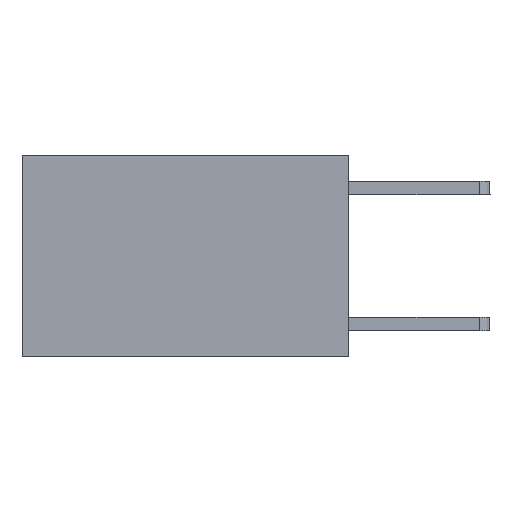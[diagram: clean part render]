
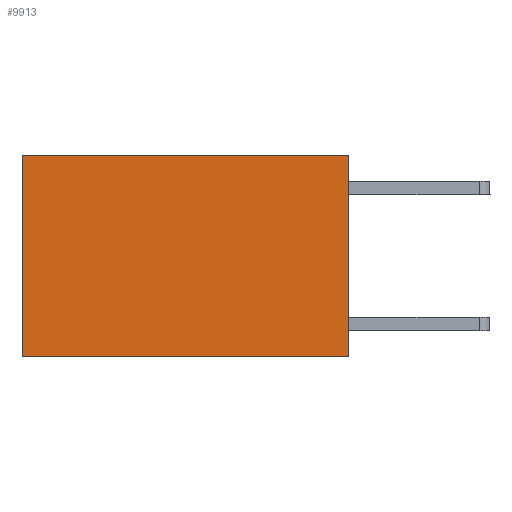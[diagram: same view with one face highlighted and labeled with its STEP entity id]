
A CAD part, left-side view. The second image highlights one B-rep face of the part: STEP entity #9913.
In plain terms, the highlighted planar face has unit normal (-1, 0, 0).
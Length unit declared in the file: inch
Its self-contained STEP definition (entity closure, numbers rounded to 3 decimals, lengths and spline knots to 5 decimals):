
#93 = LINE ( 'NONE', #1786, #122 ) ;
#122 = VECTOR ( 'NONE', #9171, 39.37008 ) ;
#345 = EDGE_CURVE ( 'NONE', #6390, #7943, #980, .T. ) ;
#445 = EDGE_CURVE ( 'NONE', #7943, #3313, #699, .T. ) ;
#623 = EDGE_CURVE ( 'NONE', #8956, #3313, #93, .T. ) ;
#664 = VECTOR ( 'NONE', #1453, 39.37008 ) ;
#699 = LINE ( 'NONE', #6083, #664 ) ;
#959 = VECTOR ( 'NONE', #5688, 39.37008 ) ;
#980 = LINE ( 'NONE', #7719, #959 ) ;
#1453 = DIRECTION ( 'NONE',  ( 0., 1., 0. ) ) ;
#1756 = CARTESIAN_POINT ( 'NONE',  ( 0.2625, 0.6, -0.37 ) ) ;
#1786 = CARTESIAN_POINT ( 'NONE',  ( 0.2625, 0.6, 0. ) ) ;
#2009 = AXIS2_PLACEMENT_3D ( 'NONE', #7611, #9934, #5160 ) ;
#2753 = ORIENTED_EDGE ( 'NONE', *, *, #345, .F. ) ;
#3242 = ORIENTED_EDGE ( 'NONE', *, *, #623, .T. ) ;
#3313 = VERTEX_POINT ( 'NONE', #1756 ) ;
#4189 = DIRECTION ( 'NONE',  ( 0., 1., 0. ) ) ;
#4450 = ORIENTED_EDGE ( 'NONE', *, *, #5101, .T. ) ;
#5101 = EDGE_CURVE ( 'NONE', #6390, #8956, #8676, .T. ) ;
#5160 = DIRECTION ( 'NONE',  ( 0., 0., -1. ) ) ;
#5546 = CARTESIAN_POINT ( 'NONE',  ( 0.2625, 0., -0.37 ) ) ;
#5688 = DIRECTION ( 'NONE',  ( 0., 0., -1. ) ) ;
#6083 = CARTESIAN_POINT ( 'NONE',  ( 0.2625, 0., -0.37 ) ) ;
#6390 = VERTEX_POINT ( 'NONE', #10628 ) ;
#7322 = CARTESIAN_POINT ( 'NONE',  ( 0.2625, 0.6, 0. ) ) ;
#7611 = CARTESIAN_POINT ( 'NONE',  ( 0.2625, 0., 0. ) ) ;
#7719 = CARTESIAN_POINT ( 'NONE',  ( 0.2625, 0., 0. ) ) ;
#7785 = EDGE_LOOP ( 'NONE', ( #3242, #7990, #2753, #4450 ) ) ;
#7943 = VERTEX_POINT ( 'NONE', #5546 ) ;
#7990 = ORIENTED_EDGE ( 'NONE', *, *, #445, .F. ) ;
#8676 = LINE ( 'NONE', #9849, #9740 ) ;
#8956 = VERTEX_POINT ( 'NONE', #7322 ) ;
#9171 = DIRECTION ( 'NONE',  ( 0., 0., -1. ) ) ;
#9740 = VECTOR ( 'NONE', #4189, 39.37008 ) ;
#9849 = CARTESIAN_POINT ( 'NONE',  ( 0.2625, 0., 0. ) ) ;
#9912 = FACE_OUTER_BOUND ( 'NONE', #7785, .T. ) ;
#9913 = ADVANCED_FACE ( 'NONE', ( #9912 ), #10611, .F. ) ;
#9934 = DIRECTION ( 'NONE',  ( 1., 0., 0. ) ) ;
#10611 = PLANE ( 'NONE',  #2009 ) ;
#10628 = CARTESIAN_POINT ( 'NONE',  ( 0.2625, 0., 0. ) ) ;
